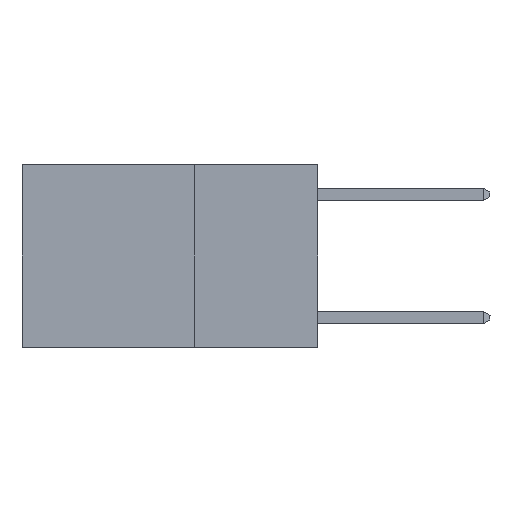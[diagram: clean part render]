
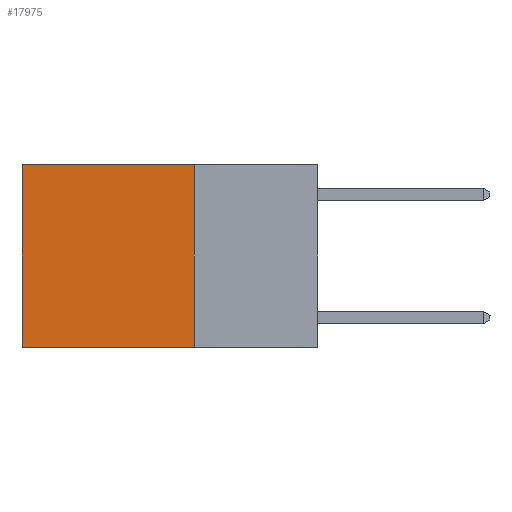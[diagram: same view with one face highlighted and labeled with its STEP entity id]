
A CAD part, left-side view. The second image highlights one B-rep face of the part: STEP entity #17975.
In plain terms, the highlighted planar face has unit normal (-1, 0, 0).
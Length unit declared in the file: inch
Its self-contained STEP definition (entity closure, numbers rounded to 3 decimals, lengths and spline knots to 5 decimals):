
#1309 = DIRECTION ( 'NONE',  ( 0., 0., -1. ) ) ;
#1521 = LINE ( 'NONE', #26904, #25158 ) ;
#1891 = VECTOR ( 'NONE', #24154, 39.37008 ) ;
#2017 = ORIENTED_EDGE ( 'NONE', *, *, #3773, .T. ) ;
#3557 = CARTESIAN_POINT ( 'NONE',  ( 0.2625, 0.25, 0. ) ) ;
#3769 = VERTEX_POINT ( 'NONE', #17378 ) ;
#3773 = EDGE_CURVE ( 'NONE', #21656, #3769, #20167, .T. ) ;
#4298 = DIRECTION ( 'NONE',  ( 1., 0., 0. ) ) ;
#5618 = CARTESIAN_POINT ( 'NONE',  ( 0.2625, 0.25, 0. ) ) ;
#6339 = VECTOR ( 'NONE', #7966, 39.37008 ) ;
#6390 = ORIENTED_EDGE ( 'NONE', *, *, #8047, .F. ) ;
#6624 = DIRECTION ( 'NONE',  ( 0., 0., -1. ) ) ;
#7208 = EDGE_CURVE ( 'NONE', #14825, #21656, #11016, .T. ) ;
#7966 = DIRECTION ( 'NONE',  ( 0., 1., 0. ) ) ;
#8047 = EDGE_CURVE ( 'NONE', #29424, #3769, #15654, .T. ) ;
#10501 = ORIENTED_EDGE ( 'NONE', *, *, #7208, .T. ) ;
#11016 = LINE ( 'NONE', #5618, #6339 ) ;
#12456 = CARTESIAN_POINT ( 'NONE',  ( 0.2625, 0.25, -0.37 ) ) ;
#12907 = CARTESIAN_POINT ( 'NONE',  ( 0.2625, 0.25, -0.37 ) ) ;
#13438 = VECTOR ( 'NONE', #1309, 39.37008 ) ;
#13778 = CARTESIAN_POINT ( 'NONE',  ( 0.2625, 0.6, 0. ) ) ;
#14316 = FACE_OUTER_BOUND ( 'NONE', #25591, .T. ) ;
#14825 = VERTEX_POINT ( 'NONE', #3557 ) ;
#15187 = CARTESIAN_POINT ( 'NONE',  ( 0.2625, 0.6, 0. ) ) ;
#15654 = LINE ( 'NONE', #12907, #1891 ) ;
#17378 = CARTESIAN_POINT ( 'NONE',  ( 0.2625, 0.6, -0.37 ) ) ;
#17975 = ADVANCED_FACE ( 'NONE', ( #14316 ), #22478, .F. ) ;
#18031 = CARTESIAN_POINT ( 'NONE',  ( 0.2625, 0.25, 0. ) ) ;
#20167 = LINE ( 'NONE', #15187, #13438 ) ;
#20320 = DIRECTION ( 'NONE',  ( 0., 0., -1. ) ) ;
#21656 = VERTEX_POINT ( 'NONE', #13778 ) ;
#22162 = EDGE_CURVE ( 'NONE', #14825, #29424, #1521, .T. ) ;
#22478 = PLANE ( 'NONE',  #25832 ) ;
#24154 = DIRECTION ( 'NONE',  ( 0., 1., 0. ) ) ;
#25158 = VECTOR ( 'NONE', #6624, 39.37008 ) ;
#25576 = ORIENTED_EDGE ( 'NONE', *, *, #22162, .F. ) ;
#25591 = EDGE_LOOP ( 'NONE', ( #2017, #6390, #25576, #10501 ) ) ;
#25832 = AXIS2_PLACEMENT_3D ( 'NONE', #18031, #4298, #20320 ) ;
#26904 = CARTESIAN_POINT ( 'NONE',  ( 0.2625, 0.25, 0. ) ) ;
#29424 = VERTEX_POINT ( 'NONE', #12456 ) ;
